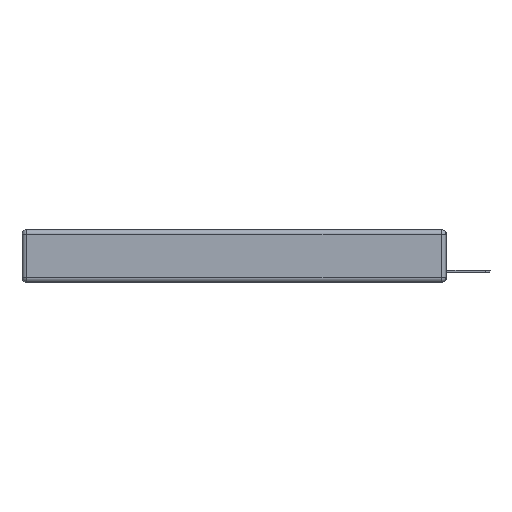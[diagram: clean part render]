
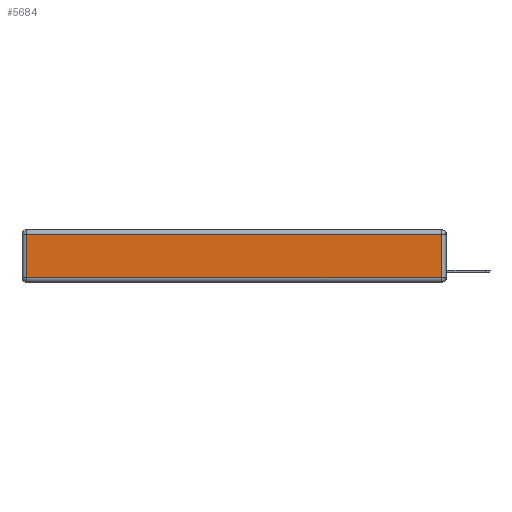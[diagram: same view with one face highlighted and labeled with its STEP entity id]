
A CAD part, left-side view. The second image highlights one B-rep face of the part: STEP entity #5684.
In plain terms, the highlighted planar face has unit normal (-1, 0, 0).
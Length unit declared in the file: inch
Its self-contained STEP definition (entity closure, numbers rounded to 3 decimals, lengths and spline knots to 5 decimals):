
#146 = ORIENTED_EDGE ( 'NONE', *, *, #8094, .T. ) ;
#728 = LINE ( 'NONE', #12190, #11075 ) ;
#1118 = CARTESIAN_POINT ( 'NONE',  ( 0., 0.03, -0.03 ) ) ;
#1214 = CARTESIAN_POINT ( 'NONE',  ( 0., 0., -0.343 ) ) ;
#1475 = CARTESIAN_POINT ( 'NONE',  ( 0., 2.72, -0.343 ) ) ;
#1531 = VERTEX_POINT ( 'NONE', #1917 ) ;
#1917 = CARTESIAN_POINT ( 'NONE',  ( 0., 0.03, -0.313 ) ) ;
#2237 = DIRECTION ( 'NONE',  ( 0., 1., 0. ) ) ;
#2604 = VECTOR ( 'NONE', #6995, 39.37008 ) ;
#2634 = ORIENTED_EDGE ( 'NONE', *, *, #5957, .T. ) ;
#2820 = ORIENTED_EDGE ( 'NONE', *, *, #9143, .T. ) ;
#3191 = VECTOR ( 'NONE', #2237, 39.37008 ) ;
#3425 = FACE_OUTER_BOUND ( 'NONE', #13884, .T. ) ;
#3616 = LINE ( 'NONE', #1475, #2604 ) ;
#5089 = ORIENTED_EDGE ( 'NONE', *, *, #13724, .T. ) ;
#5283 = LINE ( 'NONE', #14240, #14405 ) ;
#5596 = AXIS2_PLACEMENT_3D ( 'NONE', #1214, #13568, #5710 ) ;
#5684 = ADVANCED_FACE ( 'NONE', ( #3425 ), #10392, .T. ) ;
#5710 = DIRECTION ( 'NONE',  ( 0., 0., 1. ) ) ;
#5957 = EDGE_CURVE ( 'NONE', #13518, #9831, #9867, .T. ) ;
#6615 = DIRECTION ( 'NONE',  ( 0., 0., 1. ) ) ;
#6995 = DIRECTION ( 'NONE',  ( 0., 0., -1. ) ) ;
#7516 = CARTESIAN_POINT ( 'NONE',  ( 0., 2.75, -0.03 ) ) ;
#8094 = EDGE_CURVE ( 'NONE', #1531, #13518, #728, .T. ) ;
#8518 = CARTESIAN_POINT ( 'NONE',  ( 0., 2.72, -0.313 ) ) ;
#9143 = EDGE_CURVE ( 'NONE', #9831, #9246, #3616, .T. ) ;
#9246 = VERTEX_POINT ( 'NONE', #8518 ) ;
#9831 = VERTEX_POINT ( 'NONE', #14428 ) ;
#9867 = LINE ( 'NONE', #7516, #3191 ) ;
#10392 = PLANE ( 'NONE',  #5596 ) ;
#11075 = VECTOR ( 'NONE', #6615, 39.37008 ) ;
#12190 = CARTESIAN_POINT ( 'NONE',  ( 0., 0.03, -0.343 ) ) ;
#13138 = DIRECTION ( 'NONE',  ( 0., -1., 0. ) ) ;
#13518 = VERTEX_POINT ( 'NONE', #1118 ) ;
#13568 = DIRECTION ( 'NONE',  ( -1., 0., 0. ) ) ;
#13724 = EDGE_CURVE ( 'NONE', #9246, #1531, #5283, .T. ) ;
#13884 = EDGE_LOOP ( 'NONE', ( #5089, #146, #2634, #2820 ) ) ;
#14240 = CARTESIAN_POINT ( 'NONE',  ( 0., 0., -0.313 ) ) ;
#14405 = VECTOR ( 'NONE', #13138, 39.37008 ) ;
#14428 = CARTESIAN_POINT ( 'NONE',  ( 0., 2.72, -0.03 ) ) ;
